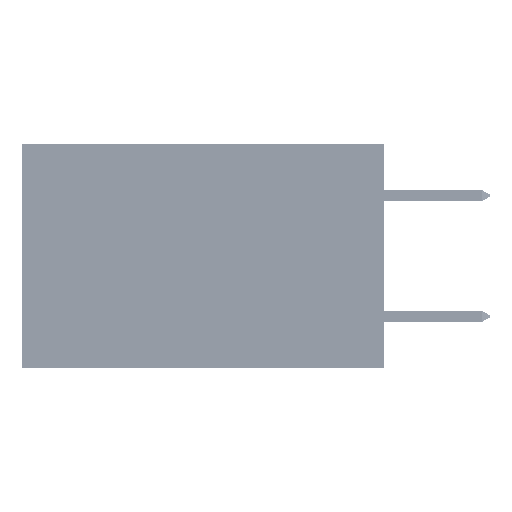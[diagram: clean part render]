
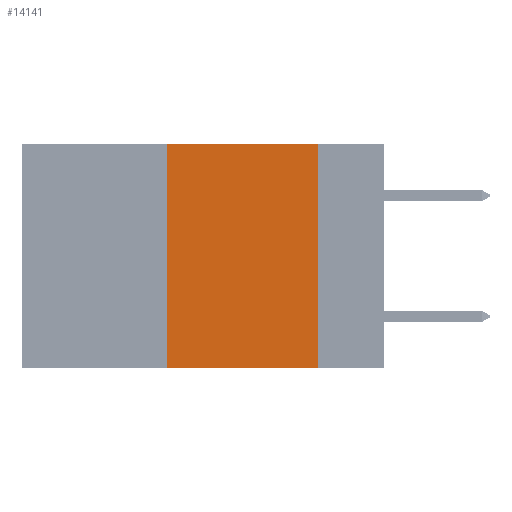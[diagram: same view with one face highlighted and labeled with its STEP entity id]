
A CAD part, left-side view. The second image highlights one B-rep face of the part: STEP entity #14141.
In plain terms, the highlighted planar face has unit normal (-1, 0, 0).
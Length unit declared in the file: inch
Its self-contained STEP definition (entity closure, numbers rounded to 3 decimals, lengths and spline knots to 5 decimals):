
#8 = CARTESIAN_POINT ( 'NONE',  ( 0., 0.11, 0. ) ) ;
#336 = ORIENTED_EDGE ( 'NONE', *, *, #28703, .F. ) ;
#1513 = DIRECTION ( 'NONE',  ( 0., -1., 0. ) ) ;
#2413 = VECTOR ( 'NONE', #1513, 39.37008 ) ;
#3507 = ORIENTED_EDGE ( 'NONE', *, *, #9732, .T. ) ;
#4088 = VERTEX_POINT ( 'NONE', #22603 ) ;
#4191 = CARTESIAN_POINT ( 'NONE',  ( 0., 0.36, 0. ) ) ;
#5402 = VERTEX_POINT ( 'NONE', #21713 ) ;
#6857 = LINE ( 'NONE', #4191, #22864 ) ;
#7191 = EDGE_LOOP ( 'NONE', ( #14675, #336, #32521, #3507 ) ) ;
#7907 = VECTOR ( 'NONE', #15030, 39.37008 ) ;
#9700 = CARTESIAN_POINT ( 'NONE',  ( 0., 0.6, 0. ) ) ;
#9732 = EDGE_CURVE ( 'NONE', #4088, #42789, #17788, .T. ) ;
#10622 = VERTEX_POINT ( 'NONE', #23398 ) ;
#14141 = ADVANCED_FACE ( 'NONE', ( #19689 ), #45470, .F. ) ;
#14675 = ORIENTED_EDGE ( 'NONE', *, *, #41319, .F. ) ;
#15030 = DIRECTION ( 'NONE',  ( 0., 0., -1. ) ) ;
#16098 = DIRECTION ( 'NONE',  ( 0., 0., 1. ) ) ;
#17788 = LINE ( 'NONE', #27939, #2413 ) ;
#19215 = CARTESIAN_POINT ( 'NONE',  ( 0., 0.11, -0.37 ) ) ;
#19231 = DIRECTION ( 'NONE',  ( 1., 0., 0. ) ) ;
#19689 = FACE_OUTER_BOUND ( 'NONE', #7191, .T. ) ;
#19995 = DIRECTION ( 'NONE',  ( 0., -1., 0. ) ) ;
#21713 = CARTESIAN_POINT ( 'NONE',  ( 0., 0.36, 0. ) ) ;
#22603 = CARTESIAN_POINT ( 'NONE',  ( 0., 0.36, -0.37 ) ) ;
#22864 = VECTOR ( 'NONE', #16098, 39.37008 ) ;
#23398 = CARTESIAN_POINT ( 'NONE',  ( 0., 0.11, 0. ) ) ;
#25877 = AXIS2_PLACEMENT_3D ( 'NONE', #45624, #19231, #42020 ) ;
#27939 = CARTESIAN_POINT ( 'NONE',  ( 0., 0.6, -0.37 ) ) ;
#28703 = EDGE_CURVE ( 'NONE', #5402, #10622, #35017, .T. ) ;
#32521 = ORIENTED_EDGE ( 'NONE', *, *, #48808, .F. ) ;
#32625 = VECTOR ( 'NONE', #19995, 39.37008 ) ;
#35017 = LINE ( 'NONE', #9700, #32625 ) ;
#39251 = LINE ( 'NONE', #8, #7907 ) ;
#41319 = EDGE_CURVE ( 'NONE', #10622, #42789, #39251, .T. ) ;
#42020 = DIRECTION ( 'NONE',  ( 0., 0., -1. ) ) ;
#42789 = VERTEX_POINT ( 'NONE', #19215 ) ;
#45470 = PLANE ( 'NONE',  #25877 ) ;
#45624 = CARTESIAN_POINT ( 'NONE',  ( 0., 0.6, 0. ) ) ;
#48808 = EDGE_CURVE ( 'NONE', #4088, #5402, #6857, .T. ) ;
